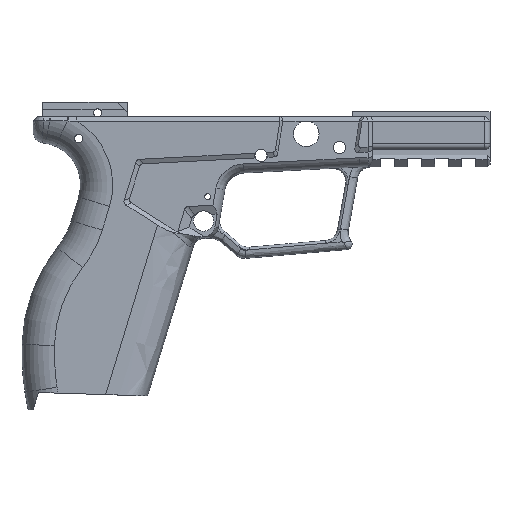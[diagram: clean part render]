
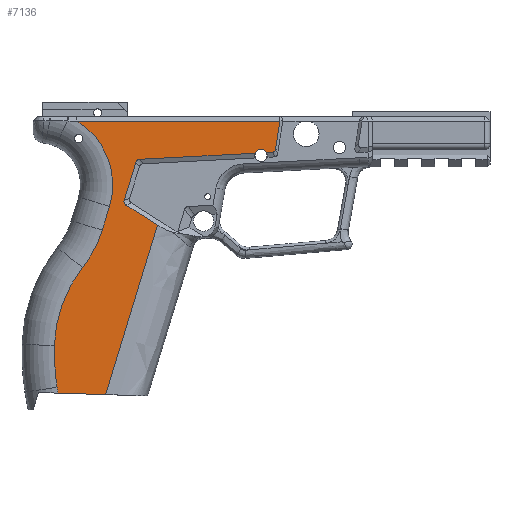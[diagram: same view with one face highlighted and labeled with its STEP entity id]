
A CAD part, left-side view. The second image highlights one B-rep face of the part: STEP entity #7136.
In plain terms, the highlighted planar face has unit normal (-1, 0, 0).
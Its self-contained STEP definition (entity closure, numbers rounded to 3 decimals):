
#132=B_SPLINE_CURVE_WITH_KNOTS('',3,(#11464,#11465,#11466,#11467),
 .UNSPECIFIED.,.F.,.F.,(4,4),(-3.646,2.394),
 .UNSPECIFIED.);
#133=B_SPLINE_CURVE_WITH_KNOTS('',3,(#11469,#11470,#11471,#11472),
 .UNSPECIFIED.,.F.,.F.,(4,4),(3.646,4.169),
 .UNSPECIFIED.);
#597=LINE('',#10899,#1323);
#666=LINE('',#11446,#1392);
#668=LINE('',#11452,#1394);
#669=LINE('',#11462,#1395);
#670=LINE('',#11474,#1396);
#671=LINE('',#11478,#1397);
#672=LINE('',#11482,#1398);
#673=LINE('',#11486,#1399);
#1323=VECTOR('',#8625,10.);
#1392=VECTOR('',#8754,10.);
#1394=VECTOR('',#8760,10.);
#1395=VECTOR('',#8769,10.);
#1396=VECTOR('',#8770,10.);
#1397=VECTOR('',#8773,10.);
#1398=VECTOR('',#8776,10.);
#1399=VECTOR('',#8779,10.);
#1788=PLANE('',#7584);
#1937=ELLIPSE('',#7590,7.191,3.);
#1938=ELLIPSE('',#7591,7.017,3.);
#1939=ELLIPSE('',#7593,4.209,2.);
#2162=FACE_OUTER_BOUND('',#2556,.T.);
#2556=EDGE_LOOP('',(#5604,#5605,#5606,#5607,#5608,#5609,#5610,#5611,#5612,
#5613,#5614,#5615,#5616,#5617,#5618,#5619,#5620,#5621,#5622));
#2875=CIRCLE('',#7585,27.5);
#2876=CIRCLE('',#7586,42.);
#2877=CIRCLE('',#7587,48.221);
#2878=CIRCLE('',#7588,89.716);
#2879=CIRCLE('',#7589,98.505);
#2880=CIRCLE('',#7592,2.25);
#3367=VERTEX_POINT('',#10896);
#3368=VERTEX_POINT('',#10898);
#3437=VERTEX_POINT('',#11445);
#3438=VERTEX_POINT('',#11449);
#3439=VERTEX_POINT('',#11451);
#3440=VERTEX_POINT('',#11453);
#3441=VERTEX_POINT('',#11455);
#3442=VERTEX_POINT('',#11457);
#3443=VERTEX_POINT('',#11459);
#3444=VERTEX_POINT('',#11461);
#3445=VERTEX_POINT('',#11463);
#3446=VERTEX_POINT('',#11468);
#3447=VERTEX_POINT('',#11473);
#3448=VERTEX_POINT('',#11475);
#3449=VERTEX_POINT('',#11477);
#3450=VERTEX_POINT('',#11479);
#3451=VERTEX_POINT('',#11481);
#3452=VERTEX_POINT('',#11483);
#3453=VERTEX_POINT('',#11485);
#4154=EDGE_CURVE('',#3367,#3368,#597,.T.);
#4256=EDGE_CURVE('',#3437,#3368,#666,.T.);
#4258=EDGE_CURVE('',#3438,#3367,#2875,.T.);
#4259=EDGE_CURVE('',#3439,#3438,#668,.T.);
#4260=EDGE_CURVE('',#3440,#3439,#2876,.T.);
#4261=EDGE_CURVE('',#3441,#3440,#2877,.T.);
#4262=EDGE_CURVE('',#3442,#3441,#2878,.T.);
#4263=EDGE_CURVE('',#3443,#3442,#2879,.T.);
#4264=EDGE_CURVE('',#3443,#3444,#669,.T.);
#4265=EDGE_CURVE('',#3445,#3444,#132,.T.);
#4266=EDGE_CURVE('',#3445,#3446,#133,.T.);
#4267=EDGE_CURVE('',#3446,#3447,#670,.T.);
#4268=EDGE_CURVE('',#3448,#3447,#1937,.T.);
#4269=EDGE_CURVE('',#3448,#3449,#671,.T.);
#4270=EDGE_CURVE('',#3450,#3449,#1938,.T.);
#4271=EDGE_CURVE('',#3450,#3451,#672,.T.);
#4272=EDGE_CURVE('',#3451,#3452,#2880,.T.);
#4273=EDGE_CURVE('',#3452,#3453,#673,.T.);
#4274=EDGE_CURVE('',#3437,#3453,#1939,.T.);
#5604=ORIENTED_EDGE('',*,*,#4154,.F.);
#5605=ORIENTED_EDGE('',*,*,#4258,.F.);
#5606=ORIENTED_EDGE('',*,*,#4259,.F.);
#5607=ORIENTED_EDGE('',*,*,#4260,.F.);
#5608=ORIENTED_EDGE('',*,*,#4261,.F.);
#5609=ORIENTED_EDGE('',*,*,#4262,.F.);
#5610=ORIENTED_EDGE('',*,*,#4263,.F.);
#5611=ORIENTED_EDGE('',*,*,#4264,.T.);
#5612=ORIENTED_EDGE('',*,*,#4265,.F.);
#5613=ORIENTED_EDGE('',*,*,#4266,.T.);
#5614=ORIENTED_EDGE('',*,*,#4267,.T.);
#5615=ORIENTED_EDGE('',*,*,#4268,.F.);
#5616=ORIENTED_EDGE('',*,*,#4269,.T.);
#5617=ORIENTED_EDGE('',*,*,#4270,.F.);
#5618=ORIENTED_EDGE('',*,*,#4271,.T.);
#5619=ORIENTED_EDGE('',*,*,#4272,.T.);
#5620=ORIENTED_EDGE('',*,*,#4273,.T.);
#5621=ORIENTED_EDGE('',*,*,#4274,.F.);
#5622=ORIENTED_EDGE('',*,*,#4256,.T.);
#7136=ADVANCED_FACE('',(#2162),#1788,.F.);
#7584=AXIS2_PLACEMENT_3D('',#11448,#8756,#8757);
#7585=AXIS2_PLACEMENT_3D('',#11450,#8758,#8759);
#7586=AXIS2_PLACEMENT_3D('',#11454,#8761,#8762);
#7587=AXIS2_PLACEMENT_3D('',#11456,#8763,#8764);
#7588=AXIS2_PLACEMENT_3D('',#11458,#8765,#8766);
#7589=AXIS2_PLACEMENT_3D('',#11460,#8767,#8768);
#7590=AXIS2_PLACEMENT_3D('',#11476,#8771,#8772);
#7591=AXIS2_PLACEMENT_3D('',#11480,#8774,#8775);
#7592=AXIS2_PLACEMENT_3D('',#11484,#8777,#8778);
#7593=AXIS2_PLACEMENT_3D('',#11487,#8780,#8781);
#8625=DIRECTION('',(0.,-1.,0.));
#8754=DIRECTION('',(0.,-0.156,0.988));
#8756=DIRECTION('center_axis',(1.,0.,0.));
#8757=DIRECTION('ref_axis',(0.,1.,0.));
#8758=DIRECTION('center_axis',(-1.,0.,0.));
#8759=DIRECTION('ref_axis',(0.,-0.853,0.522));
#8760=DIRECTION('',(0.,-0.292,0.956));
#8761=DIRECTION('center_axis',(-1.,0.,0.));
#8762=DIRECTION('ref_axis',(0.,-0.885,-0.465));
#8763=DIRECTION('center_axis',(1.,0.,0.));
#8764=DIRECTION('ref_axis',(0.,0.94,0.341));
#8765=DIRECTION('center_axis',(1.,0.,0.));
#8766=DIRECTION('ref_axis',(0.,0.998,-0.062));
#8767=DIRECTION('center_axis',(1.,0.,0.));
#8768=DIRECTION('ref_axis',(0.,0.984,-0.178));
#8769=DIRECTION('',(0.,-1.,-0.031));
#8770=DIRECTION('',(0.,0.845,0.535));
#8771=DIRECTION('center_axis',(-1.,0.,0.));
#8772=DIRECTION('ref_axis',(0.,0.938,-0.348));
#8773=DIRECTION('',(0.,-0.292,0.956));
#8774=DIRECTION('center_axis',(-1.,0.,0.));
#8775=DIRECTION('ref_axis',(0.,0.616,0.788));
#8776=DIRECTION('',(0.,-0.999,0.052));
#8777=DIRECTION('center_axis',(1.,0.,0.));
#8778=DIRECTION('ref_axis',(0.,-1.,0.));
#8779=DIRECTION('',(0.,-0.999,0.052));
#8780=DIRECTION('center_axis',(1.,0.,0.));
#8781=DIRECTION('ref_axis',(0.,-0.402,-0.916));
#10896=CARTESIAN_POINT('',(-15.125,68.451,86.));
#10898=CARTESIAN_POINT('',(-15.125,-6.762,86.));
#10899=CARTESIAN_POINT('',(-15.125,43.308,86.));
#11445=CARTESIAN_POINT('',(-15.125,-5.136,75.729));
#11446=CARTESIAN_POINT('',(-15.125,-1.434,52.36));
#11448=CARTESIAN_POINT('Origin',(-15.125,2.116,33.29));
#11449=CARTESIAN_POINT('',(-15.125,56.317,54.388));
#11450=CARTESIAN_POINT('Origin',(-15.125,82.616,62.429));
#11451=CARTESIAN_POINT('',(-15.125,59.011,45.577));
#11452=CARTESIAN_POINT('',(-15.125,59.214,44.913));
#11453=CARTESIAN_POINT('',(-15.125,66.274,31.751));
#11454=CARTESIAN_POINT('Origin',(-15.125,99.176,57.856));
#11455=CARTESIAN_POINT('',(-15.125,76.705,2.957));
#11456=CARTESIAN_POINT('Origin',(-15.125,28.499,1.78));
#11457=CARTESIAN_POINT('',(-15.125,75.74,-12.541));
#11458=CARTESIAN_POINT('Origin',(-15.125,-12.983,0.767));
#11459=CARTESIAN_POINT('',(-15.125,75.39,-14.705));
#11460=CARTESIAN_POINT('Origin',(-15.125,-21.675,2.071));
#11461=CARTESIAN_POINT('',(-15.125,57.743,-15.261));
#11462=CARTESIAN_POINT('',(-15.125,42.207,-15.75));
#11463=CARTESIAN_POINT('',(-15.125,40.084,42.5));
#11464=CARTESIAN_POINT('Ctrl Pts',(-15.125,40.084,42.5));
#11465=CARTESIAN_POINT('Ctrl Pts',(-15.125,45.97,23.246));
#11466=CARTESIAN_POINT('Ctrl Pts',(-15.125,51.856,3.993));
#11467=CARTESIAN_POINT('Ctrl Pts',(-15.125,57.743,-15.261));
#11468=CARTESIAN_POINT('',(-15.125,38.555,47.5));
#11469=CARTESIAN_POINT('Ctrl Pts',(-15.125,40.084,42.5));
#11470=CARTESIAN_POINT('Ctrl Pts',(-15.125,39.574,44.167));
#11471=CARTESIAN_POINT('Ctrl Pts',(-15.125,39.065,45.833));
#11472=CARTESIAN_POINT('Ctrl Pts',(-15.125,38.555,47.5));
#11473=CARTESIAN_POINT('',(-15.125,50.264,54.908));
#11474=CARTESIAN_POINT('',(-15.125,28.672,41.247));
#11475=CARTESIAN_POINT('',(-15.125,50.896,56.614));
#11476=CARTESIAN_POINT('Origin',(-15.125,44.155,58.143));
#11477=CARTESIAN_POINT('',(-15.125,46.568,70.773));
#11478=CARTESIAN_POINT('',(-15.125,49.754,60.35));
#11479=CARTESIAN_POINT('',(-15.125,45.212,71.832));
#11480=CARTESIAN_POINT('Origin',(-15.125,41.751,66.005));
#11481=CARTESIAN_POINT('',(-15.125,2.342,74.079));
#11482=CARTESIAN_POINT('',(-15.125,-20.801,75.292));
#11483=CARTESIAN_POINT('',(-15.125,-1.744,74.293));
#11484=CARTESIAN_POINT('Origin',(-15.125,0.25,73.25));
#11485=CARTESIAN_POINT('',(-15.125,-4.028,74.413));
#11486=CARTESIAN_POINT('',(-15.125,-20.801,75.292));
#11487=CARTESIAN_POINT('Origin',(-15.125,-2.687,78.348));
